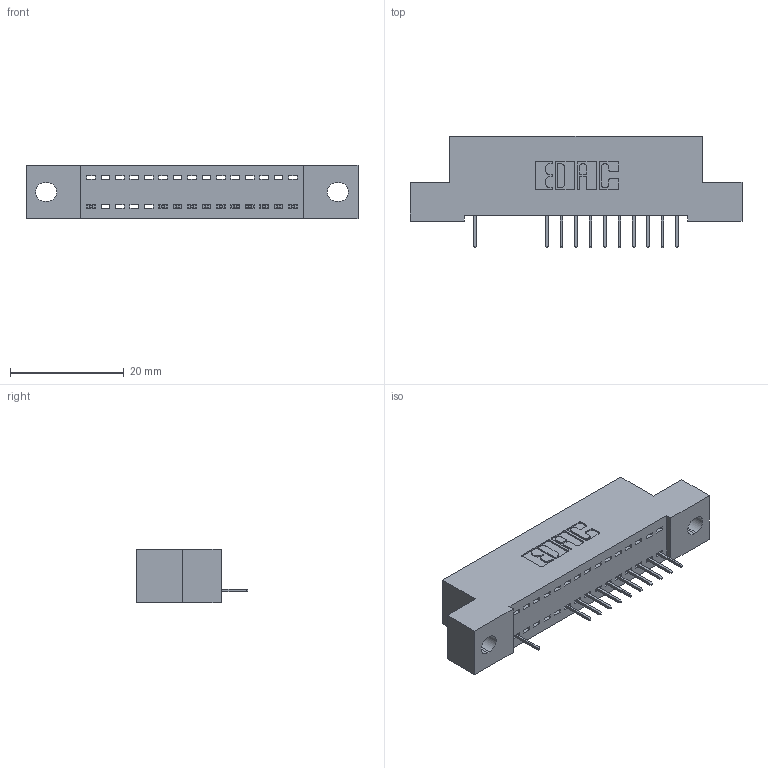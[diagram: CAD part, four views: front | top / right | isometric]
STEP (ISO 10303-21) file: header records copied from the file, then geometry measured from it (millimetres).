
FILE_DESCRIPTION (( 'STEP AP203' ), '1' );
FILE_NAME ('392-015-524-102.STEP', '2018-08-15T00:53:23', ( '' ), ( '' ), 'SwSTEP 2.0', 'SolidWorks 2016', '' );
FILE_SCHEMA (( 'CONFIG_CONTROL_DESIGN' ));
Length unit declared in the file: inch
Products named in the file (3): 342 Part_.128 Slot; 345-292-001_345-293-124; 392-015-524-102
Assembly tree (12 placements, depth 2):
  392-015-524-102
    342 Part_.128 Slot
    345-292-001_345-293-124  x11
Bounding box: 58.42 x 19.69 x 9.4 mm (x, y, z)
Volume: 4881.5 mm3; surface area: 6051.7 mm2
Topology: 12 solids, 12 shells, 844 faces, 2459 edges, 1594 vertices
Faces by surface type: plane 646, cylinder 198
Entity records: 12611 total; most frequent: CARTESIAN_POINT 2203, ORIENTED_EDGE 2158, DIRECTION 1909, EDGE_CURVE 1079, VECTOR 955, LINE 955, VERTEX_POINT 714, AXIS2_PLACEMENT_3D 477
